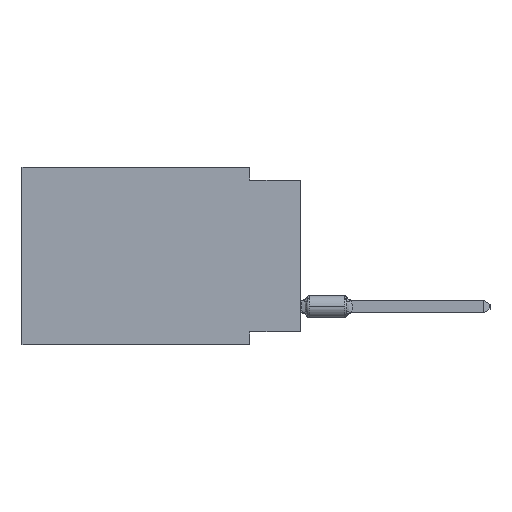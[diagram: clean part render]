
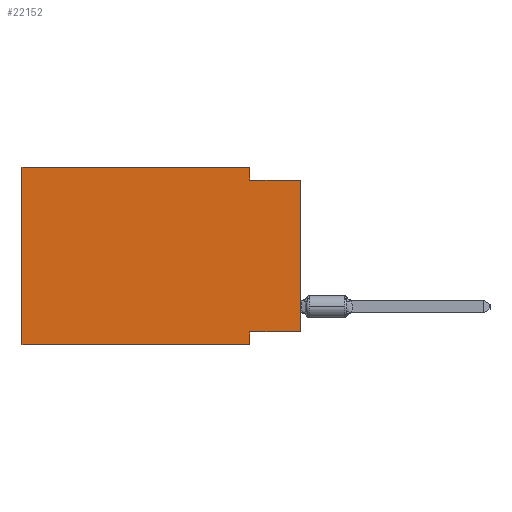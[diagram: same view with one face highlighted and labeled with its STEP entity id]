
A CAD part, left-side view. The second image highlights one B-rep face of the part: STEP entity #22152.
In plain terms, the highlighted planar face has unit normal (-1, 0, 0).
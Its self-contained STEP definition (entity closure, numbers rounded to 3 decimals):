
#532 = LINE ( 'NONE', #9994, #8806 ) ;
#678 = FACE_OUTER_BOUND ( 'NONE', #14945, .T. ) ;
#689 = LINE ( 'NONE', #15908, #8850 ) ;
#751 = VERTEX_POINT ( 'NONE', #3648 ) ;
#781 = CARTESIAN_POINT ( 'NONE',  ( 0., 13.97, 0. ) ) ;
#869 = CARTESIAN_POINT ( 'NONE',  ( 0., 2.54, 0. ) ) ;
#1281 = LINE ( 'NONE', #8780, #9691 ) ;
#1491 = VERTEX_POINT ( 'NONE', #20533 ) ;
#1560 = EDGE_CURVE ( 'NONE', #751, #15216, #20302, .T. ) ;
#3231 = CARTESIAN_POINT ( 'NONE',  ( 0., 0., -0.635 ) ) ;
#3648 = CARTESIAN_POINT ( 'NONE',  ( 0., 2.54, -0.635 ) ) ;
#3951 = VECTOR ( 'NONE', #16730, 1000. ) ;
#4414 = VERTEX_POINT ( 'NONE', #781 ) ;
#4797 = VERTEX_POINT ( 'NONE', #869 ) ;
#4949 = ORIENTED_EDGE ( 'NONE', *, *, #9117, .F. ) ;
#5248 = ORIENTED_EDGE ( 'NONE', *, *, #14489, .T. ) ;
#6210 = CARTESIAN_POINT ( 'NONE',  ( 0., 0., 0. ) ) ;
#7330 = EDGE_CURVE ( 'NONE', #10118, #1491, #1281, .T. ) ;
#8213 = CARTESIAN_POINT ( 'NONE',  ( 0., 2.54, 0. ) ) ;
#8274 = CARTESIAN_POINT ( 'NONE',  ( 0., 2.54, -8.255 ) ) ;
#8690 = VECTOR ( 'NONE', #16864, 1000. ) ;
#8780 = CARTESIAN_POINT ( 'NONE',  ( 0., 13.97, -8.89 ) ) ;
#8806 = VECTOR ( 'NONE', #13557, 1000. ) ;
#8850 = VECTOR ( 'NONE', #19589, 1000. ) ;
#9117 = EDGE_CURVE ( 'NONE', #4797, #751, #15941, .T. ) ;
#9691 = VECTOR ( 'NONE', #12461, 1000. ) ;
#9994 = CARTESIAN_POINT ( 'NONE',  ( 0., 0., -8.255 ) ) ;
#10118 = VERTEX_POINT ( 'NONE', #12434 ) ;
#10205 = ORIENTED_EDGE ( 'NONE', *, *, #18520, .F. ) ;
#10871 = LINE ( 'NONE', #14683, #15640 ) ;
#10944 = EDGE_CURVE ( 'NONE', #10118, #4414, #10871, .T. ) ;
#11334 = LINE ( 'NONE', #20783, #8690 ) ;
#12224 = VERTEX_POINT ( 'NONE', #8274 ) ;
#12434 = CARTESIAN_POINT ( 'NONE',  ( 0., 13.97, -8.89 ) ) ;
#12461 = DIRECTION ( 'NONE',  ( 0., -1., 0. ) ) ;
#13557 = DIRECTION ( 'NONE',  ( 0., 1., 0. ) ) ;
#13737 = VECTOR ( 'NONE', #15662, 1000. ) ;
#14180 = ORIENTED_EDGE ( 'NONE', *, *, #19610, .F. ) ;
#14489 = EDGE_CURVE ( 'NONE', #20320, #15216, #23467, .T. ) ;
#14683 = CARTESIAN_POINT ( 'NONE',  ( 0., 13.97, 0. ) ) ;
#14945 = EDGE_LOOP ( 'NONE', ( #5248, #21604, #4949, #14180, #18391, #21055, #23374, #10205 ) ) ;
#15216 = VERTEX_POINT ( 'NONE', #16826 ) ;
#15640 = VECTOR ( 'NONE', #18474, 1000. ) ;
#15662 = DIRECTION ( 'NONE',  ( 0., 0., 1. ) ) ;
#15908 = CARTESIAN_POINT ( 'NONE',  ( 0., 2.54, -8.89 ) ) ;
#15941 = LINE ( 'NONE', #8213, #15961 ) ;
#15961 = VECTOR ( 'NONE', #19264, 1000. ) ;
#16730 = DIRECTION ( 'NONE',  ( 0., -1., 0. ) ) ;
#16789 = CARTESIAN_POINT ( 'NONE',  ( 0., 0., -8.255 ) ) ;
#16826 = CARTESIAN_POINT ( 'NONE',  ( 0., 0., -0.635 ) ) ;
#16864 = DIRECTION ( 'NONE',  ( 0., -1., 0. ) ) ;
#16998 = PLANE ( 'NONE',  #21667 ) ;
#17504 = DIRECTION ( 'NONE',  ( 0., 0., -1. ) ) ;
#18391 = ORIENTED_EDGE ( 'NONE', *, *, #10944, .F. ) ;
#18474 = DIRECTION ( 'NONE',  ( 0., 0., 1. ) ) ;
#18520 = EDGE_CURVE ( 'NONE', #20320, #12224, #532, .T. ) ;
#19264 = DIRECTION ( 'NONE',  ( 0., 0., -1. ) ) ;
#19589 = DIRECTION ( 'NONE',  ( 0., 0., -1. ) ) ;
#19610 = EDGE_CURVE ( 'NONE', #4414, #4797, #11334, .T. ) ;
#20302 = LINE ( 'NONE', #3231, #3951 ) ;
#20320 = VERTEX_POINT ( 'NONE', #16789 ) ;
#20533 = CARTESIAN_POINT ( 'NONE',  ( 0., 2.54, -8.89 ) ) ;
#20783 = CARTESIAN_POINT ( 'NONE',  ( 0., 13.97, 0. ) ) ;
#21055 = ORIENTED_EDGE ( 'NONE', *, *, #7330, .T. ) ;
#21604 = ORIENTED_EDGE ( 'NONE', *, *, #1560, .F. ) ;
#21667 = AXIS2_PLACEMENT_3D ( 'NONE', #23114, #22613, #17504 ) ;
#22152 = ADVANCED_FACE ( 'NONE', ( #678 ), #16998, .F. ) ;
#22613 = DIRECTION ( 'NONE',  ( 1., 0., 0. ) ) ;
#23114 = CARTESIAN_POINT ( 'NONE',  ( 0., 13.97, 0. ) ) ;
#23374 = ORIENTED_EDGE ( 'NONE', *, *, #24208, .F. ) ;
#23467 = LINE ( 'NONE', #6210, #13737 ) ;
#24208 = EDGE_CURVE ( 'NONE', #12224, #1491, #689, .T. ) ;
